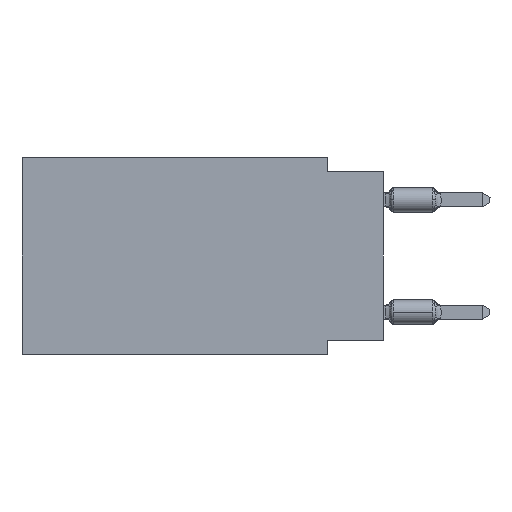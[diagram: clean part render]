
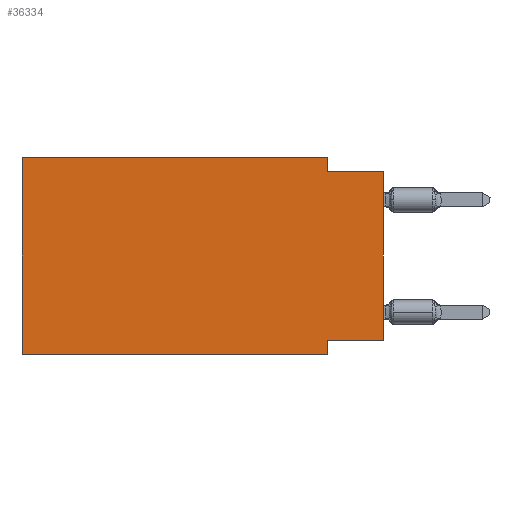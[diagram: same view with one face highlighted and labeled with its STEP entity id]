
A CAD part, left-side view. The second image highlights one B-rep face of the part: STEP entity #36334.
In plain terms, the highlighted planar face has unit normal (-1, 0, 0).
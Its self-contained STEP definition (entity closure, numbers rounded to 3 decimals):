
#496 = VERTEX_POINT ( 'NONE', #17367 ) ;
#504 = DIRECTION ( 'NONE',  ( 1., 0., 0. ) ) ;
#634 = ORIENTED_EDGE ( 'NONE', *, *, #27738, .F. ) ;
#788 = ORIENTED_EDGE ( 'NONE', *, *, #33602, .F. ) ;
#837 = LINE ( 'NONE', #15135, #23169 ) ;
#847 = VECTOR ( 'NONE', #4825, 1000. ) ;
#1473 = EDGE_CURVE ( 'NONE', #496, #13574, #15226, .T. ) ;
#1715 = ORIENTED_EDGE ( 'NONE', *, *, #1473, .F. ) ;
#3300 = CARTESIAN_POINT ( 'NONE',  ( 0., 16.383, 0. ) ) ;
#3332 = ORIENTED_EDGE ( 'NONE', *, *, #30736, .T. ) ;
#3376 = CARTESIAN_POINT ( 'NONE',  ( 0., 0., 0. ) ) ;
#3770 = CARTESIAN_POINT ( 'NONE',  ( 0., 0., -8.255 ) ) ;
#4071 = EDGE_CURVE ( 'NONE', #6029, #29311, #20265, .T. ) ;
#4814 = CARTESIAN_POINT ( 'NONE',  ( 0., 16.383, 0. ) ) ;
#4825 = DIRECTION ( 'NONE',  ( 0., 0., 1. ) ) ;
#5419 = VECTOR ( 'NONE', #31743, 1000. ) ;
#5886 = EDGE_LOOP ( 'NONE', ( #32453, #27561, #1715, #27432, #11612, #3332, #788, #634 ) ) ;
#6029 = VERTEX_POINT ( 'NONE', #3770 ) ;
#6122 = VERTEX_POINT ( 'NONE', #9899 ) ;
#7228 = DIRECTION ( 'NONE',  ( 0., -1., 0. ) ) ;
#7708 = CARTESIAN_POINT ( 'NONE',  ( 0., 0., -0.635 ) ) ;
#8314 = FACE_OUTER_BOUND ( 'NONE', #5886, .T. ) ;
#9216 = VECTOR ( 'NONE', #23891, 1000. ) ;
#9899 = CARTESIAN_POINT ( 'NONE',  ( 0., 16.383, 0. ) ) ;
#10019 = DIRECTION ( 'NONE',  ( 0., -1., 0. ) ) ;
#10208 = LINE ( 'NONE', #21882, #36252 ) ;
#11236 = CARTESIAN_POINT ( 'NONE',  ( 0., 2.54, -8.89 ) ) ;
#11612 = ORIENTED_EDGE ( 'NONE', *, *, #16327, .F. ) ;
#13574 = VERTEX_POINT ( 'NONE', #19277 ) ;
#15135 = CARTESIAN_POINT ( 'NONE',  ( 0., 16.383, -8.89 ) ) ;
#15226 = LINE ( 'NONE', #18196, #5419 ) ;
#16140 = DIRECTION ( 'NONE',  ( 0., 0., 1. ) ) ;
#16327 = EDGE_CURVE ( 'NONE', #29906, #6122, #30227, .T. ) ;
#17217 = PLANE ( 'NONE',  #32837 ) ;
#17367 = CARTESIAN_POINT ( 'NONE',  ( 0., 2.54, 0. ) ) ;
#17727 = EDGE_CURVE ( 'NONE', #13574, #29311, #10208, .T. ) ;
#18196 = CARTESIAN_POINT ( 'NONE',  ( 0., 2.54, 0. ) ) ;
#19047 = CARTESIAN_POINT ( 'NONE',  ( 0., 2.54, -8.89 ) ) ;
#19106 = CARTESIAN_POINT ( 'NONE',  ( 0., 16.383, 0. ) ) ;
#19277 = CARTESIAN_POINT ( 'NONE',  ( 0., 2.54, -0.635 ) ) ;
#19984 = VECTOR ( 'NONE', #16140, 1000. ) ;
#20265 = LINE ( 'NONE', #3376, #847 ) ;
#20267 = VECTOR ( 'NONE', #32953, 1000. ) ;
#20528 = DIRECTION ( 'NONE',  ( 0., -1., 0. ) ) ;
#20888 = VERTEX_POINT ( 'NONE', #24709 ) ;
#21882 = CARTESIAN_POINT ( 'NONE',  ( 0., 0., -0.635 ) ) ;
#21963 = CARTESIAN_POINT ( 'NONE',  ( 0., 16.383, -8.89 ) ) ;
#22371 = LINE ( 'NONE', #19047, #20267 ) ;
#23029 = LINE ( 'NONE', #19106, #31790 ) ;
#23169 = VECTOR ( 'NONE', #20528, 1000. ) ;
#23891 = DIRECTION ( 'NONE',  ( 0., 1., 0. ) ) ;
#24709 = CARTESIAN_POINT ( 'NONE',  ( 0., 2.54, -8.255 ) ) ;
#26838 = LINE ( 'NONE', #29075, #9216 ) ;
#27432 = ORIENTED_EDGE ( 'NONE', *, *, #29062, .F. ) ;
#27561 = ORIENTED_EDGE ( 'NONE', *, *, #17727, .F. ) ;
#27738 = EDGE_CURVE ( 'NONE', #6029, #20888, #26838, .T. ) ;
#29062 = EDGE_CURVE ( 'NONE', #6122, #496, #23029, .T. ) ;
#29075 = CARTESIAN_POINT ( 'NONE',  ( 0., 0., -8.255 ) ) ;
#29311 = VERTEX_POINT ( 'NONE', #7708 ) ;
#29906 = VERTEX_POINT ( 'NONE', #21963 ) ;
#30227 = LINE ( 'NONE', #4814, #19984 ) ;
#30736 = EDGE_CURVE ( 'NONE', #29906, #33859, #837, .T. ) ;
#31743 = DIRECTION ( 'NONE',  ( 0., 0., -1. ) ) ;
#31790 = VECTOR ( 'NONE', #10019, 1000. ) ;
#32453 = ORIENTED_EDGE ( 'NONE', *, *, #4071, .T. ) ;
#32837 = AXIS2_PLACEMENT_3D ( 'NONE', #3300, #504, #33914 ) ;
#32953 = DIRECTION ( 'NONE',  ( 0., 0., -1. ) ) ;
#33602 = EDGE_CURVE ( 'NONE', #20888, #33859, #22371, .T. ) ;
#33859 = VERTEX_POINT ( 'NONE', #11236 ) ;
#33914 = DIRECTION ( 'NONE',  ( 0., 0., -1. ) ) ;
#36252 = VECTOR ( 'NONE', #7228, 1000. ) ;
#36334 = ADVANCED_FACE ( 'NONE', ( #8314 ), #17217, .F. ) ;
